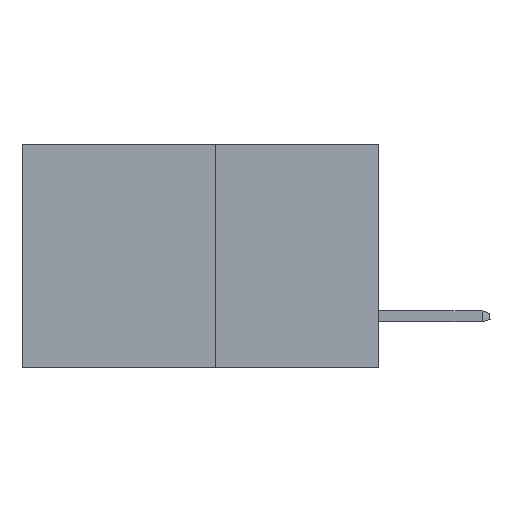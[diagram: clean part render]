
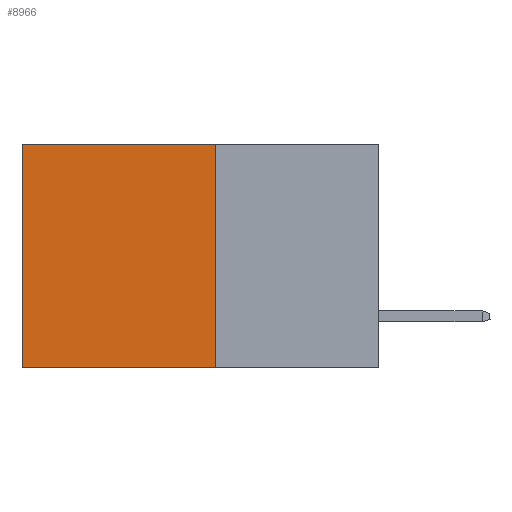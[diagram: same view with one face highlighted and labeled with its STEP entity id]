
A CAD part, left-side view. The second image highlights one B-rep face of the part: STEP entity #8966.
In plain terms, the highlighted planar face has unit normal (-1, 0, 0).
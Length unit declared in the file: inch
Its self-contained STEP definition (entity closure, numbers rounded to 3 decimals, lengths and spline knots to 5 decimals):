
#158 = DIRECTION ( 'NONE',  ( 0., 1., 0. ) ) ;
#1074 = VECTOR ( 'NONE', #4670, 39.37008 ) ;
#1823 = VERTEX_POINT ( 'NONE', #13727 ) ;
#2042 = VERTEX_POINT ( 'NONE', #3595 ) ;
#2495 = VECTOR ( 'NONE', #158, 39.37008 ) ;
#2825 = DIRECTION ( 'NONE',  ( 0., 1., 0. ) ) ;
#3595 = CARTESIAN_POINT ( 'NONE',  ( 0.277, 0.27, 0. ) ) ;
#3867 = CARTESIAN_POINT ( 'NONE',  ( 0.277, 0.27, 0. ) ) ;
#4338 = DIRECTION ( 'NONE',  ( 0., 0., -1. ) ) ;
#4606 = CARTESIAN_POINT ( 'NONE',  ( 0.277, 0.27, -0.37 ) ) ;
#4670 = DIRECTION ( 'NONE',  ( 0., 0., -1. ) ) ;
#4816 = EDGE_CURVE ( 'NONE', #2042, #5949, #5757, .T. ) ;
#5014 = DIRECTION ( 'NONE',  ( 1., 0., 0. ) ) ;
#5757 = LINE ( 'NONE', #4606, #8699 ) ;
#5949 = VERTEX_POINT ( 'NONE', #8635 ) ;
#6619 = CARTESIAN_POINT ( 'NONE',  ( 0.277, 0.59, 0. ) ) ;
#6975 = LINE ( 'NONE', #12133, #1074 ) ;
#7542 = FACE_OUTER_BOUND ( 'NONE', #13557, .T. ) ;
#8635 = CARTESIAN_POINT ( 'NONE',  ( 0.277, 0.27, -0.37 ) ) ;
#8699 = VECTOR ( 'NONE', #4338, 39.37008 ) ;
#8813 = EDGE_CURVE ( 'NONE', #15274, #1823, #6975, .T. ) ;
#8966 = ADVANCED_FACE ( 'NONE', ( #7542 ), #9975, .F. ) ;
#9173 = CARTESIAN_POINT ( 'NONE',  ( 0.277, 0.27, -0.37 ) ) ;
#9196 = LINE ( 'NONE', #3867, #2495 ) ;
#9549 = LINE ( 'NONE', #9173, #12449 ) ;
#9975 = PLANE ( 'NONE',  #12231 ) ;
#11210 = ORIENTED_EDGE ( 'NONE', *, *, #8813, .T. ) ;
#11216 = CARTESIAN_POINT ( 'NONE',  ( 0.277, 0.27, -0.37 ) ) ;
#11583 = ORIENTED_EDGE ( 'NONE', *, *, #13176, .F. ) ;
#11970 = ORIENTED_EDGE ( 'NONE', *, *, #12291, .T. ) ;
#12133 = CARTESIAN_POINT ( 'NONE',  ( 0.277, 0.59, -0.37 ) ) ;
#12231 = AXIS2_PLACEMENT_3D ( 'NONE', #11216, #5014, #13704 ) ;
#12291 = EDGE_CURVE ( 'NONE', #2042, #15274, #9196, .T. ) ;
#12449 = VECTOR ( 'NONE', #2825, 39.37008 ) ;
#13176 = EDGE_CURVE ( 'NONE', #5949, #1823, #9549, .T. ) ;
#13557 = EDGE_LOOP ( 'NONE', ( #11210, #11583, #14884, #11970 ) ) ;
#13704 = DIRECTION ( 'NONE',  ( 0., 0., -1. ) ) ;
#13727 = CARTESIAN_POINT ( 'NONE',  ( 0.277, 0.59, -0.37 ) ) ;
#14884 = ORIENTED_EDGE ( 'NONE', *, *, #4816, .F. ) ;
#15274 = VERTEX_POINT ( 'NONE', #6619 ) ;
